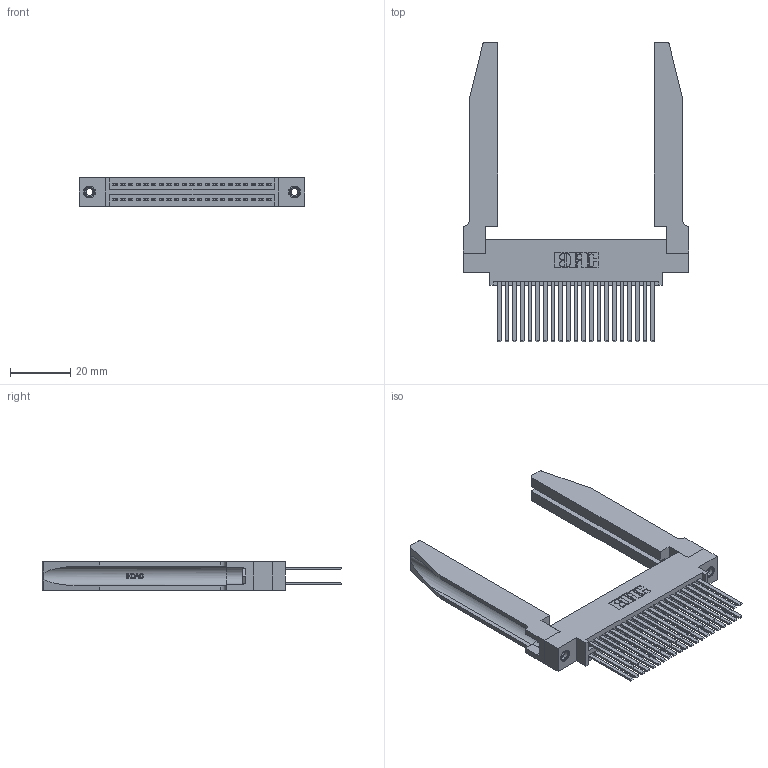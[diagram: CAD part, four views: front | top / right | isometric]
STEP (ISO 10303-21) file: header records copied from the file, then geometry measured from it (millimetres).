
FILE_DESCRIPTION (( 'STEP AP203' ), '1' );
FILE_NAME ('395-042-544-878.STEP', '2019-10-18T07:27:04', ( '' ), ( '' ), 'SwSTEP 2.0', 'SolidWorks 2016', '' );
FILE_SCHEMA (( 'CONFIG_CONTROL_DESIGN' ));
Length unit declared in the file: inch
Products named in the file (5): 345 Part_0.170 Offset - 0.156 Dia-TH; 345-292-001_345-293-144; 345-250-001_345-250-001-102; 345-220-078_345-220-078; 395-042-544-878
Assembly tree (47 placements, depth 2):
  395-042-544-878
    345 Part_0.170 Offset - 0.156 Dia-TH
    345-292-001_345-293-144  x42
    345-250-001_345-250-001-102  x2
    345-220-078_345-220-078  x2
Bounding box: 74.57 x 99.24 x 9.4 mm (x, y, z)
Volume: 15295.1 mm3; surface area: 19423.6 mm2
Topology: 47 solids, 47 shells, 2212 faces, 6463 edges, 4242 vertices
Faces by surface type: plane 1444, cylinder 716, bspline 36, cone 12, torus 4
Entity records: 23992 total; most frequent: CARTESIAN_POINT 4959, ORIENTED_EDGE 3790, DIRECTION 3389, EDGE_CURVE 1895, VECTOR 1589, LINE 1589, VERTEX_POINT 1256, AXIS2_PLACEMENT_3D 900
